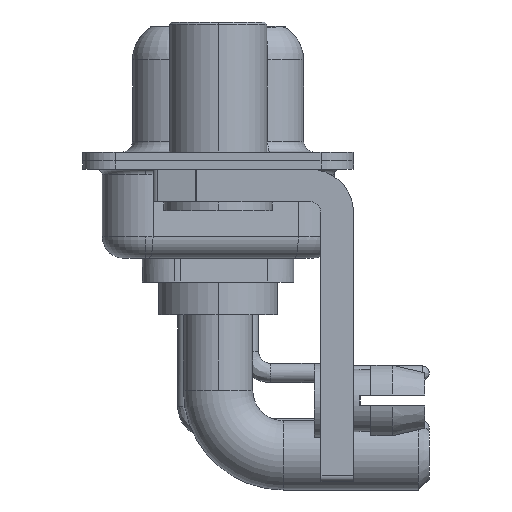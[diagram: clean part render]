
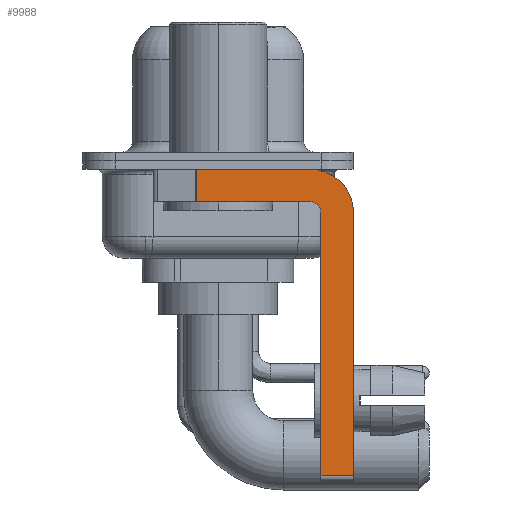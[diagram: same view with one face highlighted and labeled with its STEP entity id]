
A CAD part, left-side view. The second image highlights one B-rep face of the part: STEP entity #9988.
In plain terms, the highlighted planar face has unit normal (-1, 0, 0).
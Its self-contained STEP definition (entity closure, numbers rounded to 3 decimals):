
#1 = FACE_OUTER_BOUND ( 'NONE', #1920, .T. ) ;
#185 = VERTEX_POINT ( 'NONE', #17832 ) ;
#188 = LINE ( 'NONE', #17634, #844 ) ;
#844 = VECTOR ( 'NONE', #8250, 1000. ) ;
#1920 = EDGE_LOOP ( 'NONE', ( #19218, #17773, #2826, #4830, #19494, #12436, #2141, #8407 ) ) ;
#2141 = ORIENTED_EDGE ( 'NONE', *, *, #19217, .F. ) ;
#2455 = CIRCLE ( 'NONE', #2782, 0.5 ) ;
#2782 = AXIS2_PLACEMENT_3D ( 'NONE', #3209, #17439, #18790 ) ;
#2826 = ORIENTED_EDGE ( 'NONE', *, *, #7289, .F. ) ;
#2838 = VERTEX_POINT ( 'NONE', #6217 ) ;
#3209 = CARTESIAN_POINT ( 'NONE',  ( -2.9, -4.25, -2.4 ) ) ;
#3235 = CARTESIAN_POINT ( 'NONE',  ( -2.9, -6.25, -14.55 ) ) ;
#4126 = VERTEX_POINT ( 'NONE', #3235 ) ;
#4134 = LINE ( 'NONE', #15171, #10006 ) ;
#4273 = CARTESIAN_POINT ( 'NONE',  ( -2.9, -4.25, -1.9 ) ) ;
#4320 = AXIS2_PLACEMENT_3D ( 'NONE', #15708, #13576, #11042 ) ;
#4830 = ORIENTED_EDGE ( 'NONE', *, *, #15526, .F. ) ;
#5513 = CIRCLE ( 'NONE', #16392, 2. ) ;
#5619 = CARTESIAN_POINT ( 'NONE',  ( -2.9, 0.978, -1.9 ) ) ;
#6118 = EDGE_CURVE ( 'NONE', #12742, #14715, #5513, .T. ) ;
#6217 = CARTESIAN_POINT ( 'NONE',  ( -2.9, -4.75, -2.4 ) ) ;
#6279 = CARTESIAN_POINT ( 'NONE',  ( -2.9, -4.25, -2.4 ) ) ;
#6684 = EDGE_CURVE ( 'NONE', #10925, #2838, #11710, .T. ) ;
#7289 = EDGE_CURVE ( 'NONE', #16702, #185, #18390, .T. ) ;
#8250 = DIRECTION ( 'NONE',  ( 0., 0., -1. ) ) ;
#8407 = ORIENTED_EDGE ( 'NONE', *, *, #6118, .F. ) ;
#8433 = CARTESIAN_POINT ( 'NONE',  ( -2.9, 0.978, -0.4 ) ) ;
#8504 = EDGE_CURVE ( 'NONE', #10925, #4126, #12105, .T. ) ;
#8626 = DIRECTION ( 'NONE',  ( 0., 0., 1. ) ) ;
#8874 = VECTOR ( 'NONE', #18181, 1000. ) ;
#8982 = DIRECTION ( 'NONE',  ( 0., -1., 0. ) ) ;
#9988 = ADVANCED_FACE ( 'NONE', ( #1 ), #16670, .F. ) ;
#10006 = VECTOR ( 'NONE', #8982, 1000. ) ;
#10925 = VERTEX_POINT ( 'NONE', #11413 ) ;
#11042 = DIRECTION ( 'NONE',  ( 0., 0., -1. ) ) ;
#11156 = VERTEX_POINT ( 'NONE', #8433 ) ;
#11401 = CARTESIAN_POINT ( 'NONE',  ( -2.9, -6.25, -2.4 ) ) ;
#11413 = CARTESIAN_POINT ( 'NONE',  ( -2.9, -4.75, -14.55 ) ) ;
#11710 = LINE ( 'NONE', #19465, #19364 ) ;
#11884 = DIRECTION ( 'NONE',  ( 0., 1., 0. ) ) ;
#12105 = LINE ( 'NONE', #16853, #8874 ) ;
#12436 = ORIENTED_EDGE ( 'NONE', *, *, #8504, .T. ) ;
#12742 = VERTEX_POINT ( 'NONE', #13970 ) ;
#13172 = DIRECTION ( 'NONE',  ( 0., 0., -1. ) ) ;
#13576 = DIRECTION ( 'NONE',  ( 1., 0., 0. ) ) ;
#13641 = VECTOR ( 'NONE', #13172, 1000. ) ;
#13956 = CARTESIAN_POINT ( 'NONE',  ( -2.9, -4.25, -1.9 ) ) ;
#13970 = CARTESIAN_POINT ( 'NONE',  ( -2.9, -4.25, -0.4 ) ) ;
#14715 = VERTEX_POINT ( 'NONE', #11401 ) ;
#15171 = CARTESIAN_POINT ( 'NONE',  ( -2.9, 3., -0.4 ) ) ;
#15526 = EDGE_CURVE ( 'NONE', #2838, #16702, #2455, .T. ) ;
#15708 = CARTESIAN_POINT ( 'NONE',  ( -2.9, -4.25, -2.4 ) ) ;
#16054 = EDGE_CURVE ( 'NONE', #11156, #185, #19362, .T. ) ;
#16095 = DIRECTION ( 'NONE',  ( 0., 0., -1. ) ) ;
#16392 = AXIS2_PLACEMENT_3D ( 'NONE', #6279, #18969, #16095 ) ;
#16670 = PLANE ( 'NONE',  #4320 ) ;
#16702 = VERTEX_POINT ( 'NONE', #13956 ) ;
#16853 = CARTESIAN_POINT ( 'NONE',  ( -2.9, -4.25, -14.55 ) ) ;
#17121 = EDGE_CURVE ( 'NONE', #11156, #12742, #4134, .T. ) ;
#17439 = DIRECTION ( 'NONE',  ( -1., 0., 0. ) ) ;
#17634 = CARTESIAN_POINT ( 'NONE',  ( -2.9, -6.25, -2.4 ) ) ;
#17773 = ORIENTED_EDGE ( 'NONE', *, *, #16054, .T. ) ;
#17832 = CARTESIAN_POINT ( 'NONE',  ( -2.9, 0.978, -1.9 ) ) ;
#18067 = VECTOR ( 'NONE', #11884, 1000. ) ;
#18181 = DIRECTION ( 'NONE',  ( 0., -1., 0. ) ) ;
#18390 = LINE ( 'NONE', #4273, #18067 ) ;
#18790 = DIRECTION ( 'NONE',  ( 0., 0., 1. ) ) ;
#18969 = DIRECTION ( 'NONE',  ( 1., 0., 0. ) ) ;
#19217 = EDGE_CURVE ( 'NONE', #14715, #4126, #188, .T. ) ;
#19218 = ORIENTED_EDGE ( 'NONE', *, *, #17121, .F. ) ;
#19362 = LINE ( 'NONE', #5619, #13641 ) ;
#19364 = VECTOR ( 'NONE', #8626, 1000. ) ;
#19465 = CARTESIAN_POINT ( 'NONE',  ( -2.9, -4.75, -14.8 ) ) ;
#19494 = ORIENTED_EDGE ( 'NONE', *, *, #6684, .F. ) ;
